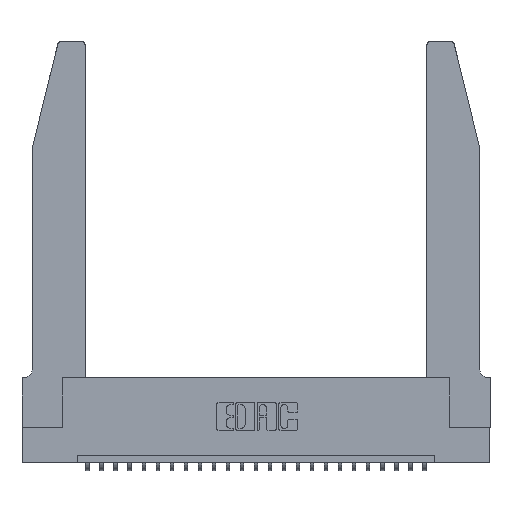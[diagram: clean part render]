
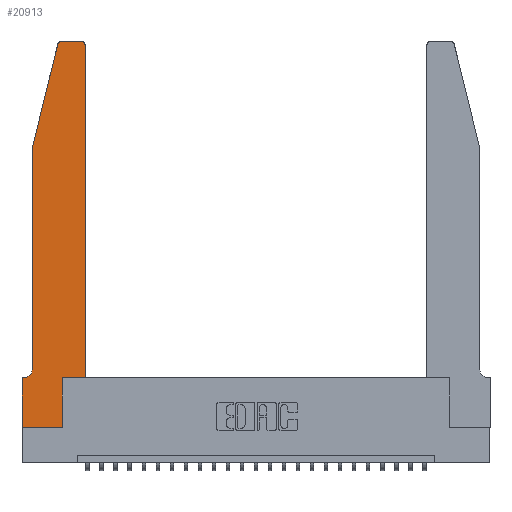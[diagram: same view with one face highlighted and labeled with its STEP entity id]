
A CAD part, top view. The second image highlights one B-rep face of the part: STEP entity #20913.
In plain terms, the highlighted planar face has unit normal (0, 0, 1).
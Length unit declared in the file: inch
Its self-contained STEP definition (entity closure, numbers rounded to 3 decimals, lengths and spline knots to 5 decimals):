
#77 = VERTEX_POINT ( 'NONE', #16881 ) ;
#465 = DIRECTION ( 'NONE',  ( -1., 0., 0. ) ) ;
#1259 = VERTEX_POINT ( 'NONE', #2275 ) ;
#1768 = AXIS2_PLACEMENT_3D ( 'NONE', #25763, #23740, #18033 ) ;
#2000 = EDGE_CURVE ( 'NONE', #22343, #12949, #14522, .T. ) ;
#2191 = PLANE ( 'NONE',  #19221 ) ;
#2237 = EDGE_CURVE ( 'NONE', #1259, #23912, #12972, .T. ) ;
#2275 = CARTESIAN_POINT ( 'NONE',  ( 0.4505, 2.72, 0.37 ) ) ;
#2395 = VERTEX_POINT ( 'NONE', #24509 ) ;
#2818 = DIRECTION ( 'NONE',  ( -1., 0., 0. ) ) ;
#3381 = ORIENTED_EDGE ( 'NONE', *, *, #2000, .T. ) ;
#4066 = EDGE_CURVE ( 'NONE', #18838, #5359, #22267, .T. ) ;
#4445 = ORIENTED_EDGE ( 'NONE', *, *, #15337, .T. ) ;
#4671 = LINE ( 'NONE', #20407, #21851 ) ;
#4902 = CARTESIAN_POINT ( 'NONE',  ( 0.2865, 0.35, 0.37 ) ) ;
#4983 = LINE ( 'NONE', #22217, #17516 ) ;
#5359 = VERTEX_POINT ( 'NONE', #12994 ) ;
#5742 = DIRECTION ( 'NONE',  ( 0., 1., 0. ) ) ;
#6060 = DIRECTION ( 'NONE',  ( -0.239, -0.971, 0. ) ) ;
#6337 = DIRECTION ( 'NONE',  ( 0., 1., 0. ) ) ;
#6383 = VECTOR ( 'NONE', #12001, 39.37008 ) ;
#6401 = ORIENTED_EDGE ( 'NONE', *, *, #6867, .T. ) ;
#6637 = CARTESIAN_POINT ( 'NONE',  ( 0.284, 2.75, 0.37 ) ) ;
#6867 = EDGE_CURVE ( 'NONE', #23912, #10551, #4671, .T. ) ;
#7135 = CIRCLE ( 'NONE', #13110, 0.03 ) ;
#8170 = LINE ( 'NONE', #15884, #22851 ) ;
#8504 = VERTEX_POINT ( 'NONE', #20817 ) ;
#9939 = ORIENTED_EDGE ( 'NONE', *, *, #23758, .T. ) ;
#9944 = CARTESIAN_POINT ( 'NONE',  ( 0., 0., 0.37 ) ) ;
#10100 = VECTOR ( 'NONE', #10548, 39.37008 ) ;
#10268 = CARTESIAN_POINT ( 'NONE',  ( 0.4205, 2.75, 0.37 ) ) ;
#10488 = LINE ( 'NONE', #9944, #15826 ) ;
#10548 = DIRECTION ( 'NONE',  ( 1., 0., 0. ) ) ;
#10551 = VERTEX_POINT ( 'NONE', #6637 ) ;
#10599 = ORIENTED_EDGE ( 'NONE', *, *, #19792, .T. ) ;
#10995 = VECTOR ( 'NONE', #6060, 39.37008 ) ;
#11144 = LINE ( 'NONE', #11673, #19868 ) ;
#11291 = ORIENTED_EDGE ( 'NONE', *, *, #4066, .T. ) ;
#11673 = CARTESIAN_POINT ( 'NONE',  ( 0., 0., 0.37 ) ) ;
#12001 = DIRECTION ( 'NONE',  ( 0., -1., 0. ) ) ;
#12055 = DIRECTION ( 'NONE',  ( 0., 0., 1. ) ) ;
#12204 = DIRECTION ( 'NONE',  ( 0., -1., 0. ) ) ;
#12472 = CARTESIAN_POINT ( 'NONE',  ( 0.4505, 0.35, 0.37 ) ) ;
#12615 = CARTESIAN_POINT ( 'NONE',  ( 0.0755, 0.35, 0.37 ) ) ;
#12644 = ORIENTED_EDGE ( 'NONE', *, *, #14516, .T. ) ;
#12949 = VERTEX_POINT ( 'NONE', #17008 ) ;
#12961 = EDGE_LOOP ( 'NONE', ( #6401, #12644, #25418, #14934, #3381, #15367, #4445, #10599, #9939, #11291, #17334, #15342 ) ) ;
#12972 = CIRCLE ( 'NONE', #23404, 0.03 ) ;
#12994 = CARTESIAN_POINT ( 'NONE',  ( 0.4505, 0.35, 0.37 ) ) ;
#13110 = AXIS2_PLACEMENT_3D ( 'NONE', #18002, #12055, #19990 ) ;
#13209 = EDGE_CURVE ( 'NONE', #12949, #77, #19395, .T. ) ;
#13329 = EDGE_CURVE ( 'NONE', #5359, #1259, #4983, .T. ) ;
#13514 = VERTEX_POINT ( 'NONE', #24515 ) ;
#14350 = DIRECTION ( 'NONE',  ( 0., 0., 1. ) ) ;
#14516 = EDGE_CURVE ( 'NONE', #10551, #2395, #7135, .T. ) ;
#14522 = CIRCLE ( 'NONE', #1768, 0.07 ) ;
#14898 = CARTESIAN_POINT ( 'NONE',  ( 0.0755, 2., 0.37 ) ) ;
#14934 = ORIENTED_EDGE ( 'NONE', *, *, #21216, .T. ) ;
#15337 = EDGE_CURVE ( 'NONE', #77, #13514, #10488, .T. ) ;
#15342 = ORIENTED_EDGE ( 'NONE', *, *, #2237, .T. ) ;
#15367 = ORIENTED_EDGE ( 'NONE', *, *, #13209, .T. ) ;
#15451 = CARTESIAN_POINT ( 'NONE',  ( 0.0755, 0.42, 0.37 ) ) ;
#15826 = VECTOR ( 'NONE', #12204, 39.37008 ) ;
#15884 = CARTESIAN_POINT ( 'NONE',  ( 0.2865, 0.35, 0.37 ) ) ;
#16016 = CARTESIAN_POINT ( 'NONE',  ( 0.0755, 2., 0.37 ) ) ;
#16213 = CARTESIAN_POINT ( 'NONE',  ( 0., 0.35, 0.37 ) ) ;
#16881 = CARTESIAN_POINT ( 'NONE',  ( 0., 0.35, 0.37 ) ) ;
#17008 = CARTESIAN_POINT ( 'NONE',  ( 0.0055, 0.35, 0.37 ) ) ;
#17334 = ORIENTED_EDGE ( 'NONE', *, *, #13329, .T. ) ;
#17516 = VECTOR ( 'NONE', #6337, 39.37008 ) ;
#18002 = CARTESIAN_POINT ( 'NONE',  ( 0.284, 2.72, 0.37 ) ) ;
#18033 = DIRECTION ( 'NONE',  ( -1., 0., 0. ) ) ;
#18838 = VERTEX_POINT ( 'NONE', #4902 ) ;
#19221 = AXIS2_PLACEMENT_3D ( 'NONE', #16213, #14350, #20198 ) ;
#19395 = LINE ( 'NONE', #12615, #22190 ) ;
#19779 = DIRECTION ( 'NONE',  ( 1., 0., 0. ) ) ;
#19792 = EDGE_CURVE ( 'NONE', #13514, #8504, #11144, .T. ) ;
#19868 = VECTOR ( 'NONE', #19779, 39.37008 ) ;
#19990 = DIRECTION ( 'NONE',  ( 1., 0., 0. ) ) ;
#20100 = CARTESIAN_POINT ( 'NONE',  ( 0.0755, 2., 0.37 ) ) ;
#20198 = DIRECTION ( 'NONE',  ( 1., 0., 0. ) ) ;
#20407 = CARTESIAN_POINT ( 'NONE',  ( 0.2605, 2.75, 0.37 ) ) ;
#20440 = FACE_OUTER_BOUND ( 'NONE', #12961, .T. ) ;
#20633 = CARTESIAN_POINT ( 'NONE',  ( 0.4205, 2.72, 0.37 ) ) ;
#20727 = DIRECTION ( 'NONE',  ( 0., 0., 1. ) ) ;
#20817 = CARTESIAN_POINT ( 'NONE',  ( 0.2865, 0., 0.37 ) ) ;
#20913 = ADVANCED_FACE ( 'NONE', ( #20440 ), #2191, .T. ) ;
#21216 = EDGE_CURVE ( 'NONE', #25932, #22343, #22309, .T. ) ;
#21605 = LINE ( 'NONE', #16016, #10995 ) ;
#21851 = VECTOR ( 'NONE', #465, 39.37008 ) ;
#22190 = VECTOR ( 'NONE', #2818, 39.37008 ) ;
#22217 = CARTESIAN_POINT ( 'NONE',  ( 0.4505, 0.35, 0.37 ) ) ;
#22267 = LINE ( 'NONE', #12472, #10100 ) ;
#22309 = LINE ( 'NONE', #20100, #6383 ) ;
#22343 = VERTEX_POINT ( 'NONE', #15451 ) ;
#22736 = DIRECTION ( 'NONE',  ( 1., 0., 0. ) ) ;
#22851 = VECTOR ( 'NONE', #5742, 39.37008 ) ;
#23139 = EDGE_CURVE ( 'NONE', #2395, #25932, #21605, .T. ) ;
#23404 = AXIS2_PLACEMENT_3D ( 'NONE', #20633, #20727, #22736 ) ;
#23740 = DIRECTION ( 'NONE',  ( 0., 0., -1. ) ) ;
#23758 = EDGE_CURVE ( 'NONE', #8504, #18838, #8170, .T. ) ;
#23912 = VERTEX_POINT ( 'NONE', #10268 ) ;
#24509 = CARTESIAN_POINT ( 'NONE',  ( 0.25487, 2.72718, 0.37 ) ) ;
#24515 = CARTESIAN_POINT ( 'NONE',  ( 0., 0., 0.37 ) ) ;
#25418 = ORIENTED_EDGE ( 'NONE', *, *, #23139, .T. ) ;
#25763 = CARTESIAN_POINT ( 'NONE',  ( 0.0055, 0.42, 0.37 ) ) ;
#25932 = VERTEX_POINT ( 'NONE', #14898 ) ;
